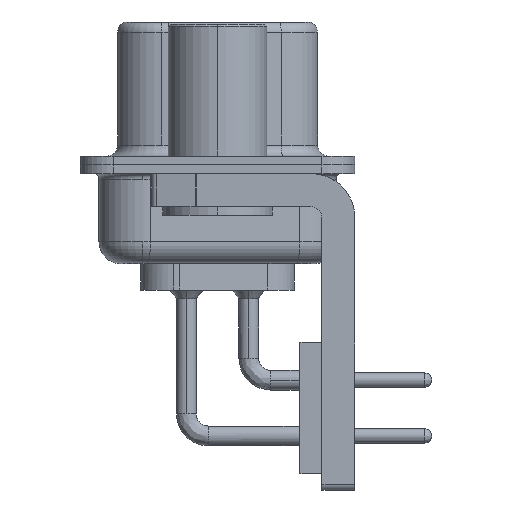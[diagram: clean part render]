
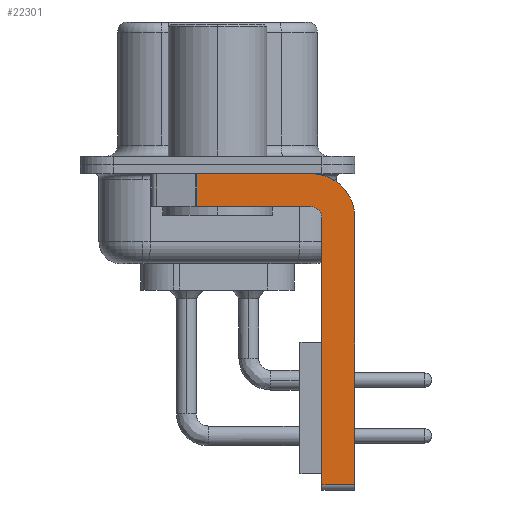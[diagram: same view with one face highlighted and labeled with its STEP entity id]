
A CAD part, left-side view. The second image highlights one B-rep face of the part: STEP entity #22301.
In plain terms, the highlighted planar face has unit normal (-1, 0, 0).
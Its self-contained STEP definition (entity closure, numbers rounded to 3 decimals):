
#247 = VECTOR ( 'NONE', #1889, 1000. ) ;
#288 = EDGE_CURVE ( 'NONE', #10008, #2698, #23011, .T. ) ;
#921 = VERTEX_POINT ( 'NONE', #3208 ) ;
#1832 = VERTEX_POINT ( 'NONE', #22934 ) ;
#1889 = DIRECTION ( 'NONE',  ( 0., 1., 0. ) ) ;
#2039 = VECTOR ( 'NONE', #3951, 1000. ) ;
#2669 = LINE ( 'NONE', #18817, #24220 ) ;
#2698 = VERTEX_POINT ( 'NONE', #24057 ) ;
#3020 = DIRECTION ( 'NONE',  ( 0., 0., 1. ) ) ;
#3049 = DIRECTION ( 'NONE',  ( -1., 0., 0. ) ) ;
#3208 = CARTESIAN_POINT ( 'NONE',  ( -2.9, -4.75, -2.4 ) ) ;
#3301 = CARTESIAN_POINT ( 'NONE',  ( -2.9, -4.25, -2.4 ) ) ;
#3358 = VERTEX_POINT ( 'NONE', #9750 ) ;
#3378 = DIRECTION ( 'NONE',  ( 1., 0., 0. ) ) ;
#3918 = VECTOR ( 'NONE', #10032, 1000. ) ;
#3951 = DIRECTION ( 'NONE',  ( 0., -1., 0. ) ) ;
#4095 = DIRECTION ( 'NONE',  ( 0., -1., 0. ) ) ;
#4314 = AXIS2_PLACEMENT_3D ( 'NONE', #21730, #10040, #23684 ) ;
#4489 = ORIENTED_EDGE ( 'NONE', *, *, #8269, .F. ) ;
#5657 = ORIENTED_EDGE ( 'NONE', *, *, #10044, .F. ) ;
#5826 = CARTESIAN_POINT ( 'NONE',  ( -2.9, -4.25, -1.9 ) ) ;
#5846 = FACE_OUTER_BOUND ( 'NONE', #15031, .T. ) ;
#7005 = DIRECTION ( 'NONE',  ( 0., 0., -1. ) ) ;
#7174 = VERTEX_POINT ( 'NONE', #15279 ) ;
#7877 = AXIS2_PLACEMENT_3D ( 'NONE', #3301, #3049, #3020 ) ;
#7911 = CARTESIAN_POINT ( 'NONE',  ( -2.9, -4.25, -14.55 ) ) ;
#8269 = EDGE_CURVE ( 'NONE', #921, #1832, #23227, .T. ) ;
#8370 = ORIENTED_EDGE ( 'NONE', *, *, #18466, .F. ) ;
#9750 = CARTESIAN_POINT ( 'NONE',  ( -2.9, 0.978, -1.9 ) ) ;
#9952 = PLANE ( 'NONE',  #4314 ) ;
#10008 = VERTEX_POINT ( 'NONE', #21649 ) ;
#10032 = DIRECTION ( 'NONE',  ( 0., 0., -1. ) ) ;
#10040 = DIRECTION ( 'NONE',  ( 1., 0., 0. ) ) ;
#10044 = EDGE_CURVE ( 'NONE', #22542, #19428, #15343, .T. ) ;
#10063 = LINE ( 'NONE', #25313, #21078 ) ;
#10077 = VECTOR ( 'NONE', #4095, 1000. ) ;
#10965 = LINE ( 'NONE', #5826, #247 ) ;
#13678 = DIRECTION ( 'NONE',  ( 0., 0., 1. ) ) ;
#14840 = EDGE_CURVE ( 'NONE', #22542, #3358, #2669, .T. ) ;
#15031 = EDGE_LOOP ( 'NONE', ( #5657, #18311, #22989, #4489, #8370, #20066, #15550, #21617 ) ) ;
#15279 = CARTESIAN_POINT ( 'NONE',  ( -2.9, -6.25, -2.4 ) ) ;
#15306 = CARTESIAN_POINT ( 'NONE',  ( -2.9, -4.25, -2.4 ) ) ;
#15343 = LINE ( 'NONE', #16013, #10077 ) ;
#15550 = ORIENTED_EDGE ( 'NONE', *, *, #24959, .F. ) ;
#16013 = CARTESIAN_POINT ( 'NONE',  ( -2.9, 3., -0.4 ) ) ;
#17293 = DIRECTION ( 'NONE',  ( 0., 0., -1. ) ) ;
#17875 = CARTESIAN_POINT ( 'NONE',  ( -2.9, -6.25, -2.4 ) ) ;
#17879 = AXIS2_PLACEMENT_3D ( 'NONE', #15306, #3378, #17293 ) ;
#18311 = ORIENTED_EDGE ( 'NONE', *, *, #14840, .T. ) ;
#18466 = EDGE_CURVE ( 'NONE', #10008, #921, #10063, .T. ) ;
#18817 = CARTESIAN_POINT ( 'NONE',  ( -2.9, 0.978, -1.9 ) ) ;
#18842 = EDGE_CURVE ( 'NONE', #19428, #7174, #23479, .T. ) ;
#18909 = CARTESIAN_POINT ( 'NONE',  ( -2.9, -4.25, -0.4 ) ) ;
#19345 = LINE ( 'NONE', #17875, #3918 ) ;
#19428 = VERTEX_POINT ( 'NONE', #18909 ) ;
#20066 = ORIENTED_EDGE ( 'NONE', *, *, #288, .T. ) ;
#20543 = EDGE_CURVE ( 'NONE', #1832, #3358, #10965, .T. ) ;
#21078 = VECTOR ( 'NONE', #13678, 1000. ) ;
#21617 = ORIENTED_EDGE ( 'NONE', *, *, #18842, .F. ) ;
#21649 = CARTESIAN_POINT ( 'NONE',  ( -2.9, -4.75, -14.55 ) ) ;
#21730 = CARTESIAN_POINT ( 'NONE',  ( -2.9, -4.25, -2.4 ) ) ;
#22301 = ADVANCED_FACE ( 'NONE', ( #5846 ), #9952, .F. ) ;
#22542 = VERTEX_POINT ( 'NONE', #24430 ) ;
#22934 = CARTESIAN_POINT ( 'NONE',  ( -2.9, -4.25, -1.9 ) ) ;
#22989 = ORIENTED_EDGE ( 'NONE', *, *, #20543, .F. ) ;
#23011 = LINE ( 'NONE', #7911, #2039 ) ;
#23227 = CIRCLE ( 'NONE', #7877, 0.5 ) ;
#23479 = CIRCLE ( 'NONE', #17879, 2. ) ;
#23684 = DIRECTION ( 'NONE',  ( 0., 0., -1. ) ) ;
#24057 = CARTESIAN_POINT ( 'NONE',  ( -2.9, -6.25, -14.55 ) ) ;
#24220 = VECTOR ( 'NONE', #7005, 1000. ) ;
#24430 = CARTESIAN_POINT ( 'NONE',  ( -2.9, 0.978, -0.4 ) ) ;
#24959 = EDGE_CURVE ( 'NONE', #7174, #2698, #19345, .T. ) ;
#25313 = CARTESIAN_POINT ( 'NONE',  ( -2.9, -4.75, -14.8 ) ) ;
